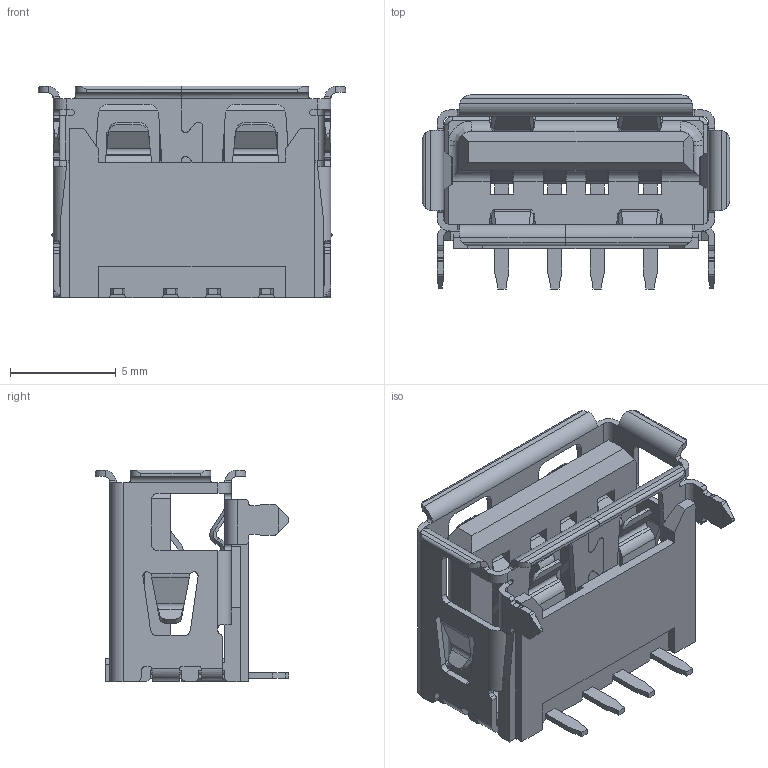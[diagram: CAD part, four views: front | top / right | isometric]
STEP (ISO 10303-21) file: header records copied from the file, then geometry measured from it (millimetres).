
FILE_DESCRIPTION (( 'STEP AP214' ), '1' );
FILE_NAME ('690A104-621-411.STEP', '2021-01-13T21:39:28', ( '' ), ( '' ), 'SwSTEP 2.0', 'SolidWorks 2020', '' );
FILE_SCHEMA (( 'AUTOMOTIVE_DESIGN' ));
Length unit declared in the file: millimetre
Products named in the file (4): 690A104-621-411; Shell 690A104-621-411; Contact 690A104-621-411; Insulator 690A104-621-411
Assembly tree (6 placements, depth 2):
  690A104-621-411
    Insulator 690A104-621-411
    Contact 690A104-621-411  x4
    Shell 690A104-621-411
Bounding box: 14.5 x 9.15 x 10 mm (x, y, z)
Volume: 327.9 mm3; surface area: 1499.1 mm2
Topology: 6 solids, 6 shells, 1256 faces, 3504 edges, 2248 vertices
Faces by surface type: plane 712, cylinder 391, bspline 137, cone 16
Entity records: 36570 total; most frequent: CARTESIAN_POINT 11789, ORIENTED_EDGE 5502, DIRECTION 4634, EDGE_CURVE 2751, LINE 1940, VECTOR 1940, VERTEX_POINT 1750, AXIS2_PLACEMENT_3D 1347
